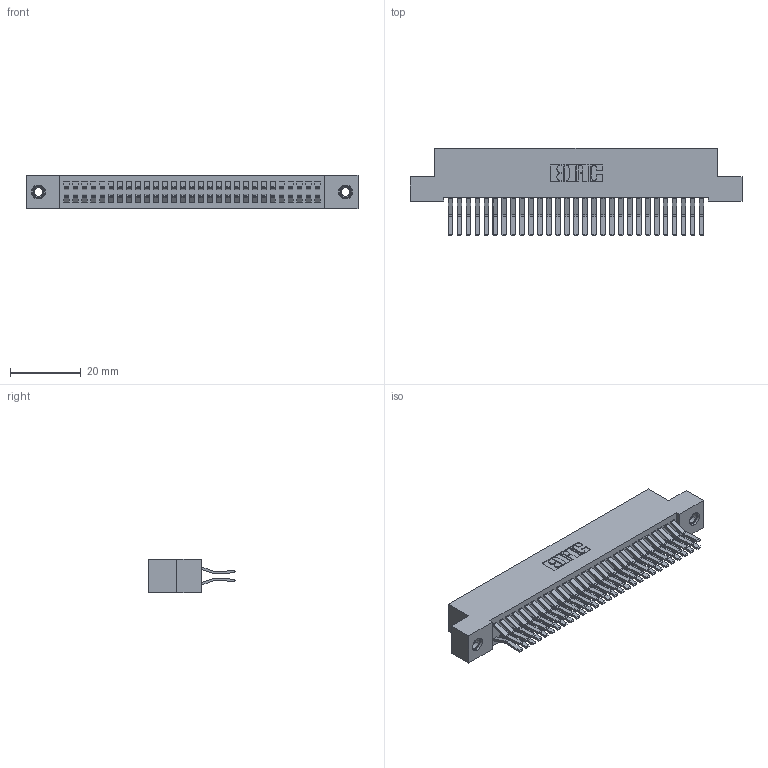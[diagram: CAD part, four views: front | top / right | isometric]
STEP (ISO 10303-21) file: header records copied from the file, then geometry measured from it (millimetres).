
FILE_DESCRIPTION (( 'STEP AP203' ), '1' );
FILE_NAME ('392-058-560-207.STEP', '2019-10-08T17:08:22', ( '' ), ( '' ), 'SwSTEP 2.0', 'SolidWorks 2016', '' );
FILE_SCHEMA (( 'CONFIG_CONTROL_DESIGN' ));
Length unit declared in the file: inch
Products named in the file (4): 342 Part_TI; 345-292-001_560 Tail; 345-250-001_345-250-005-103; 392-058-560-207
Assembly tree (61 placements, depth 2):
  392-058-560-207
    342 Part_TI
    345-292-001_560 Tail  x58
    345-250-001_345-250-005-103  x2
Bounding box: 93.98 x 24.78 x 9.4 mm (x, y, z)
Volume: 8750.7 mm3; surface area: 14862.4 mm2
Topology: 61 solids, 61 shells, 3302 faces, 9773 edges, 6430 vertices
Faces by surface type: plane 2186, cylinder 1100, cone 12, torus 4
Entity records: 21480 total; most frequent: CARTESIAN_POINT 3557, ORIENTED_EDGE 3486, DIRECTION 3097, EDGE_CURVE 1743, LINE 1591, VECTOR 1591, VERTEX_POINT 1156, AXIS2_PLACEMENT_3D 753
